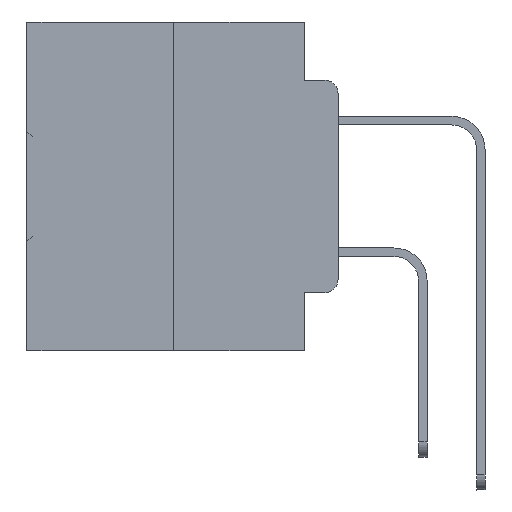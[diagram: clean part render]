
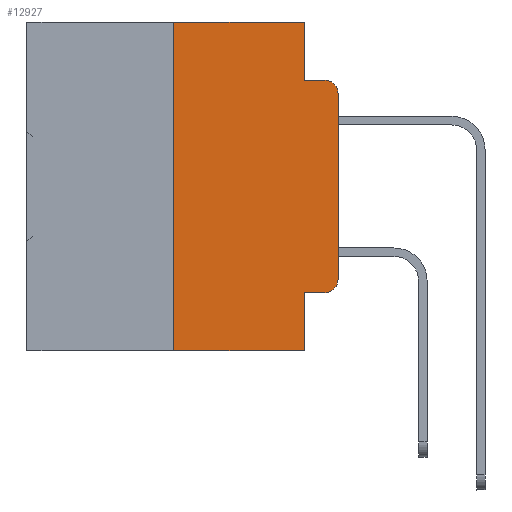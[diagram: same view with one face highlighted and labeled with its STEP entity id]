
A CAD part, left-side view. The second image highlights one B-rep face of the part: STEP entity #12927.
In plain terms, the highlighted planar face has unit normal (-1, 0, 0).
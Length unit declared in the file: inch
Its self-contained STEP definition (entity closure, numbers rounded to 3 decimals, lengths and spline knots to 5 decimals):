
#173 = EDGE_CURVE ( 'NONE', #36210, #32371, #34420, .T. ) ;
#1531 = ORIENTED_EDGE ( 'NONE', *, *, #37242, .F. ) ;
#1853 = EDGE_CURVE ( 'NONE', #14546, #31923, #8722, .T. ) ;
#2360 = DIRECTION ( 'NONE',  ( -1., 0., 0. ) ) ;
#2552 = VECTOR ( 'NONE', #28941, 39.37008 ) ;
#2640 = CARTESIAN_POINT ( 'NONE',  ( 0., 0., -0.1085 ) ) ;
#3444 = CARTESIAN_POINT ( 'NONE',  ( 0., 0.051, 0. ) ) ;
#3455 = CARTESIAN_POINT ( 'NONE',  ( 0., 0.051, 0. ) ) ;
#3812 = EDGE_CURVE ( 'NONE', #36459, #31923, #27620, .T. ) ;
#4505 = AXIS2_PLACEMENT_3D ( 'NONE', #27098, #9773, #29940 ) ;
#5455 = LINE ( 'NONE', #15996, #27658 ) ;
#5634 = ORIENTED_EDGE ( 'NONE', *, *, #31626, .F. ) ;
#5776 = EDGE_CURVE ( 'NONE', #16203, #36459, #23843, .T. ) ;
#5803 = CARTESIAN_POINT ( 'NONE',  ( 0., 0.25, 0. ) ) ;
#6278 = EDGE_CURVE ( 'NONE', #11331, #25907, #37085, .T. ) ;
#6436 = CARTESIAN_POINT ( 'NONE',  ( 0., 0.051, -0.0885 ) ) ;
#6766 = CARTESIAN_POINT ( 'NONE',  ( 0., 0.25, 0. ) ) ;
#6782 = LINE ( 'NONE', #3455, #29820 ) ;
#7001 = CARTESIAN_POINT ( 'NONE',  ( 0., 0.473, 0. ) ) ;
#7259 = DIRECTION ( 'NONE',  ( 0., 0., -1. ) ) ;
#7795 = VECTOR ( 'NONE', #29799, 39.37008 ) ;
#8465 = VECTOR ( 'NONE', #22874, 39.37008 ) ;
#8669 = LINE ( 'NONE', #26194, #24033 ) ;
#8722 = LINE ( 'NONE', #6436, #7795 ) ;
#8878 = DIRECTION ( 'NONE',  ( 0., -1., 0. ) ) ;
#8964 = AXIS2_PLACEMENT_3D ( 'NONE', #7001, #30095, #12809 ) ;
#9436 = LINE ( 'NONE', #5803, #2552 ) ;
#9773 = DIRECTION ( 'NONE',  ( -1., 0., 0. ) ) ;
#9790 = ORIENTED_EDGE ( 'NONE', *, *, #173, .F. ) ;
#11028 = EDGE_LOOP ( 'NONE', ( #11038, #31805, #25099, #1531, #9790, #5634, #30486, #24673, #16544, #26049 ) ) ;
#11038 = ORIENTED_EDGE ( 'NONE', *, *, #5776, .T. ) ;
#11245 = CARTESIAN_POINT ( 'NONE',  ( 0., 0., 0. ) ) ;
#11322 = CIRCLE ( 'NONE', #4505, 0.02 ) ;
#11331 = VERTEX_POINT ( 'NONE', #33874 ) ;
#12809 = DIRECTION ( 'NONE',  ( 0., 0., -1. ) ) ;
#12927 = ADVANCED_FACE ( 'NONE', ( #32086 ), #18534, .F. ) ;
#14092 = CARTESIAN_POINT ( 'NONE',  ( 0., 0.051, -0.0885 ) ) ;
#14546 = VERTEX_POINT ( 'NONE', #14092 ) ;
#14551 = CARTESIAN_POINT ( 'NONE',  ( 0., 0.051, -0.5 ) ) ;
#14964 = VERTEX_POINT ( 'NONE', #16091 ) ;
#15115 = DIRECTION ( 'NONE',  ( 0., 0., -1. ) ) ;
#15996 = CARTESIAN_POINT ( 'NONE',  ( 0., 0.051, 0. ) ) ;
#16091 = CARTESIAN_POINT ( 'NONE',  ( 0., 0.02, -0.4115 ) ) ;
#16203 = VERTEX_POINT ( 'NONE', #35857 ) ;
#16544 = ORIENTED_EDGE ( 'NONE', *, *, #25897, .T. ) ;
#17025 = VECTOR ( 'NONE', #22104, 39.37008 ) ;
#17113 = VERTEX_POINT ( 'NONE', #23353 ) ;
#18534 = PLANE ( 'NONE',  #8964 ) ;
#18837 = CARTESIAN_POINT ( 'NONE',  ( 0., 0.02, -0.0885 ) ) ;
#19758 = CARTESIAN_POINT ( 'NONE',  ( 0., 0.02, -0.1085 ) ) ;
#20100 = EDGE_CURVE ( 'NONE', #14964, #16203, #11322, .T. ) ;
#21626 = AXIS2_PLACEMENT_3D ( 'NONE', #19758, #2360, #22677 ) ;
#22104 = DIRECTION ( 'NONE',  ( 0., -1., 0. ) ) ;
#22677 = DIRECTION ( 'NONE',  ( 0., 0., -1. ) ) ;
#22874 = DIRECTION ( 'NONE',  ( 0., 0., 1. ) ) ;
#23353 = CARTESIAN_POINT ( 'NONE',  ( 0., 0.051, -0.4115 ) ) ;
#23843 = LINE ( 'NONE', #11245, #8465 ) ;
#24033 = VECTOR ( 'NONE', #8878, 39.37008 ) ;
#24673 = ORIENTED_EDGE ( 'NONE', *, *, #29737, .F. ) ;
#25099 = ORIENTED_EDGE ( 'NONE', *, *, #1853, .F. ) ;
#25897 = EDGE_CURVE ( 'NONE', #17113, #14964, #8669, .T. ) ;
#25907 = VERTEX_POINT ( 'NONE', #14551 ) ;
#26049 = ORIENTED_EDGE ( 'NONE', *, *, #20100, .T. ) ;
#26194 = CARTESIAN_POINT ( 'NONE',  ( 0., 0.051, -0.4115 ) ) ;
#26914 = VECTOR ( 'NONE', #36017, 39.37008 ) ;
#27098 = CARTESIAN_POINT ( 'NONE',  ( 0., 0.02, -0.3915 ) ) ;
#27620 = CIRCLE ( 'NONE', #21626, 0.02 ) ;
#27658 = VECTOR ( 'NONE', #7259, 39.37008 ) ;
#28941 = DIRECTION ( 'NONE',  ( 0., 0., 1. ) ) ;
#29737 = EDGE_CURVE ( 'NONE', #17113, #25907, #5455, .T. ) ;
#29799 = DIRECTION ( 'NONE',  ( 0., -1., 0. ) ) ;
#29820 = VECTOR ( 'NONE', #15115, 39.37008 ) ;
#29940 = DIRECTION ( 'NONE',  ( 0., 0., -1. ) ) ;
#30095 = DIRECTION ( 'NONE',  ( 1., 0., 0. ) ) ;
#30395 = CARTESIAN_POINT ( 'NONE',  ( 0., 0.473, 0. ) ) ;
#30486 = ORIENTED_EDGE ( 'NONE', *, *, #6278, .T. ) ;
#31626 = EDGE_CURVE ( 'NONE', #11331, #36210, #9436, .T. ) ;
#31805 = ORIENTED_EDGE ( 'NONE', *, *, #3812, .T. ) ;
#31923 = VERTEX_POINT ( 'NONE', #18837 ) ;
#32086 = FACE_OUTER_BOUND ( 'NONE', #11028, .T. ) ;
#32371 = VERTEX_POINT ( 'NONE', #3444 ) ;
#33559 = CARTESIAN_POINT ( 'NONE',  ( 0., 0.473, -0.5 ) ) ;
#33874 = CARTESIAN_POINT ( 'NONE',  ( 0., 0.25, -0.5 ) ) ;
#34420 = LINE ( 'NONE', #30395, #26914 ) ;
#35857 = CARTESIAN_POINT ( 'NONE',  ( 0., 0., -0.3915 ) ) ;
#36017 = DIRECTION ( 'NONE',  ( 0., -1., 0. ) ) ;
#36210 = VERTEX_POINT ( 'NONE', #6766 ) ;
#36459 = VERTEX_POINT ( 'NONE', #2640 ) ;
#37085 = LINE ( 'NONE', #33559, #17025 ) ;
#37242 = EDGE_CURVE ( 'NONE', #32371, #14546, #6782, .T. ) ;
